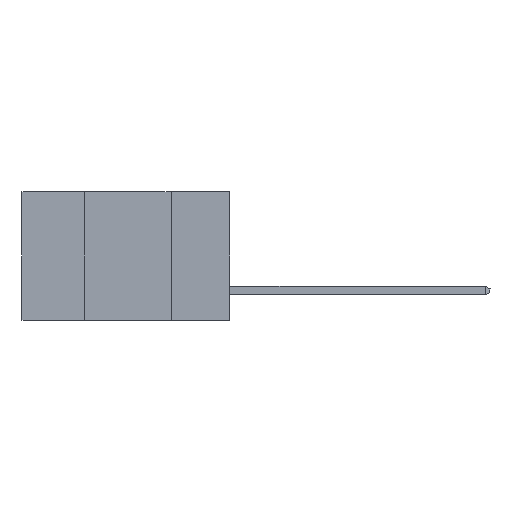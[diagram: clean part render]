
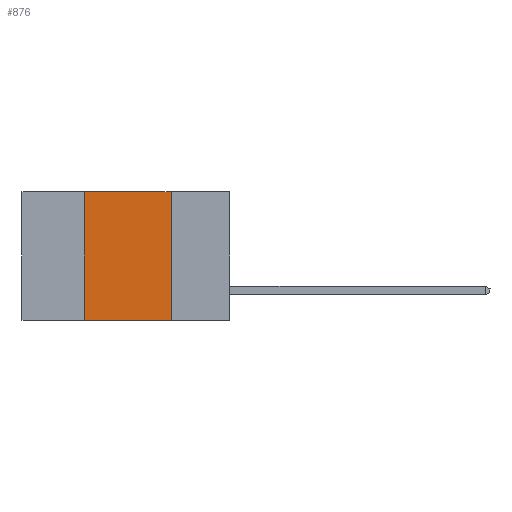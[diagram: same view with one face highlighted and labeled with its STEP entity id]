
A CAD part, left-side view. The second image highlights one B-rep face of the part: STEP entity #876.
In plain terms, the highlighted planar face has unit normal (-1, 0, 0).
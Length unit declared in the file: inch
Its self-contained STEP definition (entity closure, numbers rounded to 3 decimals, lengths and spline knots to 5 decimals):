
#195 = CARTESIAN_POINT ( 'NONE',  ( 0., 0.17, -0.37 ) ) ;
#876 = ADVANCED_FACE ( 'NONE', ( #2181 ), #6739, .F. ) ;
#1286 = EDGE_CURVE ( 'NONE', #4142, #4687, #4516, .T. ) ;
#1375 = LINE ( 'NONE', #4306, #7674 ) ;
#1612 = EDGE_CURVE ( 'NONE', #5810, #4687, #7063, .T. ) ;
#1862 = VECTOR ( 'NONE', #4331, 39.37008 ) ;
#1981 = CARTESIAN_POINT ( 'NONE',  ( 0., 0.6, -0.37 ) ) ;
#2181 = FACE_OUTER_BOUND ( 'NONE', #9207, .T. ) ;
#2252 = AXIS2_PLACEMENT_3D ( 'NONE', #4439, #3624, #2948 ) ;
#2948 = DIRECTION ( 'NONE',  ( 0., 0., -1. ) ) ;
#3288 = EDGE_CURVE ( 'NONE', #5810, #5658, #8566, .T. ) ;
#3563 = DIRECTION ( 'NONE',  ( 0., 0., 1. ) ) ;
#3624 = DIRECTION ( 'NONE',  ( 1., 0., 0. ) ) ;
#4142 = VERTEX_POINT ( 'NONE', #9358 ) ;
#4163 = VECTOR ( 'NONE', #4804, 39.37008 ) ;
#4191 = CARTESIAN_POINT ( 'NONE',  ( 0., 0.42, -0.37 ) ) ;
#4306 = CARTESIAN_POINT ( 'NONE',  ( 0., 0.6, 0. ) ) ;
#4331 = DIRECTION ( 'NONE',  ( 0., 0., -1. ) ) ;
#4439 = CARTESIAN_POINT ( 'NONE',  ( 0., 0.6, 0. ) ) ;
#4516 = LINE ( 'NONE', #7307, #1862 ) ;
#4687 = VERTEX_POINT ( 'NONE', #195 ) ;
#4804 = DIRECTION ( 'NONE',  ( 0., -1., 0. ) ) ;
#4956 = EDGE_CURVE ( 'NONE', #5658, #4142, #1375, .T. ) ;
#5203 = ORIENTED_EDGE ( 'NONE', *, *, #3288, .F. ) ;
#5545 = ORIENTED_EDGE ( 'NONE', *, *, #1612, .T. ) ;
#5658 = VERTEX_POINT ( 'NONE', #6159 ) ;
#5673 = CARTESIAN_POINT ( 'NONE',  ( 0., 0.42, -0.37 ) ) ;
#5810 = VERTEX_POINT ( 'NONE', #5673 ) ;
#6159 = CARTESIAN_POINT ( 'NONE',  ( 0., 0.42, 0. ) ) ;
#6234 = ORIENTED_EDGE ( 'NONE', *, *, #1286, .F. ) ;
#6739 = PLANE ( 'NONE',  #2252 ) ;
#6753 = ORIENTED_EDGE ( 'NONE', *, *, #4956, .F. ) ;
#6853 = VECTOR ( 'NONE', #3563, 39.37008 ) ;
#7063 = LINE ( 'NONE', #1981, #4163 ) ;
#7307 = CARTESIAN_POINT ( 'NONE',  ( 0., 0.17, -0.37 ) ) ;
#7674 = VECTOR ( 'NONE', #7809, 39.37008 ) ;
#7809 = DIRECTION ( 'NONE',  ( 0., -1., 0. ) ) ;
#8566 = LINE ( 'NONE', #4191, #6853 ) ;
#9207 = EDGE_LOOP ( 'NONE', ( #6234, #6753, #5203, #5545 ) ) ;
#9358 = CARTESIAN_POINT ( 'NONE',  ( 0., 0.17, 0. ) ) ;
